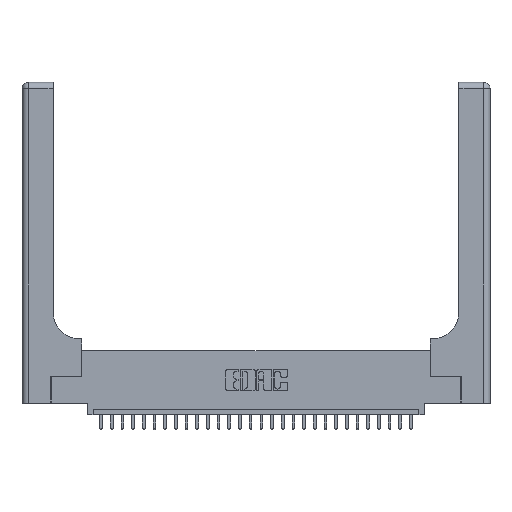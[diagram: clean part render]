
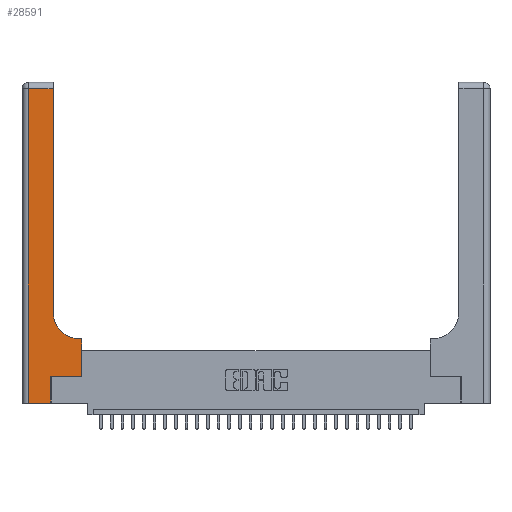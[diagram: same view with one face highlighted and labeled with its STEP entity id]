
A CAD part, top view. The second image highlights one B-rep face of the part: STEP entity #28591.
In plain terms, the highlighted planar face has unit normal (0, 0, 1).
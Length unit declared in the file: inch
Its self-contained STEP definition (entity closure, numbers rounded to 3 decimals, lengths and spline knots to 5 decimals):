
#372 = EDGE_CURVE ( 'NONE', #10911, #17649, #23315, .T. ) ;
#584 = ORIENTED_EDGE ( 'NONE', *, *, #7968, .T. ) ;
#735 = CARTESIAN_POINT ( 'NONE',  ( 0.269, 0., 0.37 ) ) ;
#1024 = DIRECTION ( 'NONE',  ( 1., 0., 0. ) ) ;
#2058 = LINE ( 'NONE', #7695, #11666 ) ;
#3406 = ORIENTED_EDGE ( 'NONE', *, *, #21714, .T. ) ;
#3416 = CARTESIAN_POINT ( 'NONE',  ( 0., 3., 0.37 ) ) ;
#3601 = CARTESIAN_POINT ( 'NONE',  ( 0.2915, 2.94, 0.37 ) ) ;
#3616 = PLANE ( 'NONE',  #6341 ) ;
#3900 = CARTESIAN_POINT ( 'NONE',  ( 0.269, 0., 0.37 ) ) ;
#5431 = VERTEX_POINT ( 'NONE', #9223 ) ;
#6124 = LINE ( 'NONE', #8599, #15752 ) ;
#6323 = ORIENTED_EDGE ( 'NONE', *, *, #14088, .T. ) ;
#6341 = AXIS2_PLACEMENT_3D ( 'NONE', #3416, #12580, #26398 ) ;
#6542 = ORIENTED_EDGE ( 'NONE', *, *, #14574, .T. ) ;
#7695 = CARTESIAN_POINT ( 'NONE',  ( 0.5585, 0.25, 0.37 ) ) ;
#7840 = CARTESIAN_POINT ( 'NONE',  ( 0., 2.94, 0.37 ) ) ;
#7882 = LINE ( 'NONE', #7840, #28293 ) ;
#7968 = EDGE_CURVE ( 'NONE', #21370, #18977, #6124, .T. ) ;
#8599 = CARTESIAN_POINT ( 'NONE',  ( 0.2915, 0.6, 0.37 ) ) ;
#8862 = ORIENTED_EDGE ( 'NONE', *, *, #372, .T. ) ;
#9211 = DIRECTION ( 'NONE',  ( 1., 0., 0. ) ) ;
#9223 = CARTESIAN_POINT ( 'NONE',  ( 0.06, 2.94, 0.37 ) ) ;
#9363 = FACE_OUTER_BOUND ( 'NONE', #17629, .T. ) ;
#9833 = CARTESIAN_POINT ( 'NONE',  ( 0.5415, 0.85, 0.37 ) ) ;
#10294 = VERTEX_POINT ( 'NONE', #24860 ) ;
#10511 = CARTESIAN_POINT ( 'NONE',  ( 0.5585, 0.25, 0.37 ) ) ;
#10709 = VERTEX_POINT ( 'NONE', #3601 ) ;
#10796 = CARTESIAN_POINT ( 'NONE',  ( 0.5415, 0.6, 0.37 ) ) ;
#10911 = VERTEX_POINT ( 'NONE', #16104 ) ;
#11119 = CARTESIAN_POINT ( 'NONE',  ( 0.06, 0., 0.37 ) ) ;
#11404 = CARTESIAN_POINT ( 'NONE',  ( 0.06, 3., 0.37 ) ) ;
#11444 = LINE ( 'NONE', #22727, #20019 ) ;
#11666 = VECTOR ( 'NONE', #12416, 39.37008 ) ;
#12416 = DIRECTION ( 'NONE',  ( 0., 1., 0. ) ) ;
#12559 = CARTESIAN_POINT ( 'NONE',  ( 0.269, 0.25, 0.37 ) ) ;
#12580 = DIRECTION ( 'NONE',  ( 0., 0., -1. ) ) ;
#12957 = VECTOR ( 'NONE', #21866, 39.37008 ) ;
#12970 = EDGE_CURVE ( 'NONE', #5431, #21805, #22458, .T. ) ;
#14088 = EDGE_CURVE ( 'NONE', #10294, #10709, #25624, .T. ) ;
#14574 = EDGE_CURVE ( 'NONE', #17649, #21370, #2058, .T. ) ;
#15752 = VECTOR ( 'NONE', #26889, 39.37008 ) ;
#15777 = DIRECTION ( 'NONE',  ( 0., -1., 0. ) ) ;
#15834 = EDGE_CURVE ( 'NONE', #18977, #10294, #22423, .T. ) ;
#16093 = VECTOR ( 'NONE', #18866, 39.37008 ) ;
#16104 = CARTESIAN_POINT ( 'NONE',  ( 0.269, 0.25, 0.37 ) ) ;
#16137 = ORIENTED_EDGE ( 'NONE', *, *, #15834, .T. ) ;
#17553 = LINE ( 'NONE', #735, #16093 ) ;
#17611 = DIRECTION ( 'NONE',  ( 0., 1., 0. ) ) ;
#17629 = EDGE_LOOP ( 'NONE', ( #6323, #3406, #20007, #22494, #21169, #8862, #6542, #584, #16137 ) ) ;
#17649 = VERTEX_POINT ( 'NONE', #10511 ) ;
#18699 = EDGE_CURVE ( 'NONE', #24870, #10911, #17553, .T. ) ;
#18866 = DIRECTION ( 'NONE',  ( 0., 1., 0. ) ) ;
#18977 = VERTEX_POINT ( 'NONE', #10796 ) ;
#19938 = CARTESIAN_POINT ( 'NONE',  ( 0.2915, 3., 0.37 ) ) ;
#20007 = ORIENTED_EDGE ( 'NONE', *, *, #12970, .T. ) ;
#20019 = VECTOR ( 'NONE', #9211, 39.37008 ) ;
#21169 = ORIENTED_EDGE ( 'NONE', *, *, #18699, .T. ) ;
#21370 = VERTEX_POINT ( 'NONE', #22171 ) ;
#21655 = DIRECTION ( 'NONE',  ( -1., 0., 0. ) ) ;
#21714 = EDGE_CURVE ( 'NONE', #10709, #5431, #7882, .T. ) ;
#21805 = VERTEX_POINT ( 'NONE', #11119 ) ;
#21866 = DIRECTION ( 'NONE',  ( 1., 0., 0. ) ) ;
#22049 = VECTOR ( 'NONE', #17611, 39.37008 ) ;
#22171 = CARTESIAN_POINT ( 'NONE',  ( 0.5585, 0.6, 0.37 ) ) ;
#22423 = CIRCLE ( 'NONE', #28244, 0.25 ) ;
#22458 = LINE ( 'NONE', #11404, #23514 ) ;
#22494 = ORIENTED_EDGE ( 'NONE', *, *, #22544, .T. ) ;
#22544 = EDGE_CURVE ( 'NONE', #21805, #24870, #11444, .T. ) ;
#22727 = CARTESIAN_POINT ( 'NONE',  ( 0., 0., 0.37 ) ) ;
#23315 = LINE ( 'NONE', #12559, #12957 ) ;
#23514 = VECTOR ( 'NONE', #15777, 39.37008 ) ;
#24860 = CARTESIAN_POINT ( 'NONE',  ( 0.2915, 0.85, 0.37 ) ) ;
#24870 = VERTEX_POINT ( 'NONE', #3900 ) ;
#25624 = LINE ( 'NONE', #19938, #22049 ) ;
#26398 = DIRECTION ( 'NONE',  ( -1., 0., 0. ) ) ;
#26889 = DIRECTION ( 'NONE',  ( -1., 0., 0. ) ) ;
#28133 = DIRECTION ( 'NONE',  ( 0., 0., -1. ) ) ;
#28244 = AXIS2_PLACEMENT_3D ( 'NONE', #9833, #28133, #1024 ) ;
#28293 = VECTOR ( 'NONE', #21655, 39.37008 ) ;
#28591 = ADVANCED_FACE ( 'NONE', ( #9363 ), #3616, .F. ) ;
